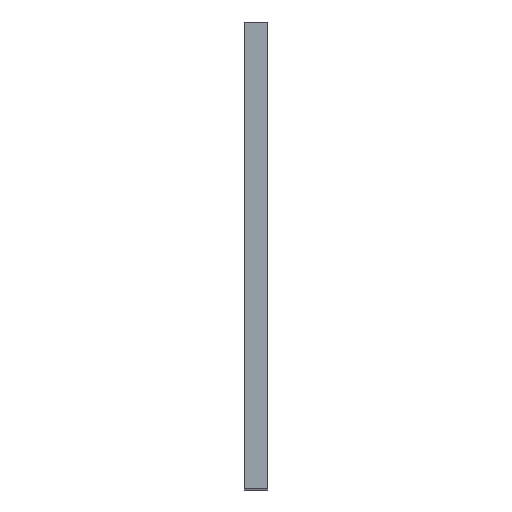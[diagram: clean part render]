
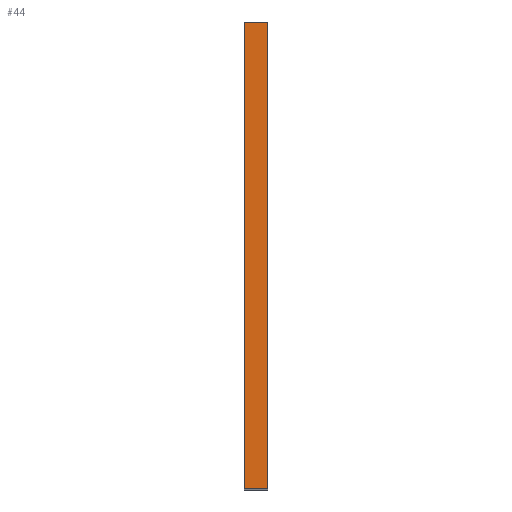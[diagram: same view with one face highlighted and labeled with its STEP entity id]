
A CAD part, top view. The second image highlights one B-rep face of the part: STEP entity #44.
In plain terms, the highlighted planar face has unit normal (0, 0, 1).
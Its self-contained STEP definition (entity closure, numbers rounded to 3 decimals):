
#23 = CARTESIAN_POINT ( 'NONE',  ( 5., 41.482, 51.853 ) ) ;
#37 = DIRECTION ( 'NONE',  ( 0., -1., 0. ) ) ;
#40 = CARTESIAN_POINT ( 'NONE',  ( 0., 0., 51.853 ) ) ;
#42 = DIRECTION ( 'NONE',  ( 0., 1., 0. ) ) ;
#44 = ADVANCED_FACE ( 'NONE', ( #452 ), #245, .F. ) ;
#46 = DIRECTION ( 'NONE',  ( 0., 0., -1. ) ) ;
#59 = DIRECTION ( 'NONE',  ( -1., 0., 0. ) ) ;
#112 = CARTESIAN_POINT ( 'NONE',  ( 0., -56.018, 51.853 ) ) ;
#222 = EDGE_CURVE ( 'NONE', #709, #799, #386, .T. ) ;
#245 = PLANE ( 'NONE',  #273 ) ;
#273 = AXIS2_PLACEMENT_3D ( 'NONE', #409, #46, #42 ) ;
#302 = LINE ( 'NONE', #510, #307 ) ;
#304 = VECTOR ( 'NONE', #635, 1000. ) ;
#307 = VECTOR ( 'NONE', #509, 1000. ) ;
#308 = VECTOR ( 'NONE', #59, 1000. ) ;
#311 = LINE ( 'NONE', #23, #308 ) ;
#313 = LINE ( 'NONE', #646, #304 ) ;
#385 = VECTOR ( 'NONE', #37, 1000. ) ;
#386 = LINE ( 'NONE', #40, #385 ) ;
#409 = CARTESIAN_POINT ( 'NONE',  ( 5., 0., 51.853 ) ) ;
#452 = FACE_OUTER_BOUND ( 'NONE', #883, .T. ) ;
#458 = EDGE_CURVE ( 'NONE', #645, #709, #311, .T. ) ;
#470 = EDGE_CURVE ( 'NONE', #696, #799, #313, .T. ) ;
#497 = EDGE_CURVE ( 'NONE', #645, #696, #302, .T. ) ;
#509 = DIRECTION ( 'NONE',  ( 0., -1., 0. ) ) ;
#510 = CARTESIAN_POINT ( 'NONE',  ( 5., 0., 51.853 ) ) ;
#594 = CARTESIAN_POINT ( 'NONE',  ( 5., 41.482, 51.853 ) ) ;
#635 = DIRECTION ( 'NONE',  ( -1., 0., 0. ) ) ;
#645 = VERTEX_POINT ( 'NONE', #594 ) ;
#646 = CARTESIAN_POINT ( 'NONE',  ( 5., -56.018, 51.853 ) ) ;
#692 = CARTESIAN_POINT ( 'NONE',  ( 0., 41.482, 51.853 ) ) ;
#695 = ORIENTED_EDGE ( 'NONE', *, *, #458, .T. ) ;
#696 = VERTEX_POINT ( 'NONE', #792 ) ;
#709 = VERTEX_POINT ( 'NONE', #692 ) ;
#728 = ORIENTED_EDGE ( 'NONE', *, *, #497, .F. ) ;
#792 = CARTESIAN_POINT ( 'NONE',  ( 5., -56.018, 51.853 ) ) ;
#799 = VERTEX_POINT ( 'NONE', #112 ) ;
#870 = ORIENTED_EDGE ( 'NONE', *, *, #222, .T. ) ;
#882 = ORIENTED_EDGE ( 'NONE', *, *, #470, .F. ) ;
#883 = EDGE_LOOP ( 'NONE', ( #870, #882, #728, #695 ) ) ;
